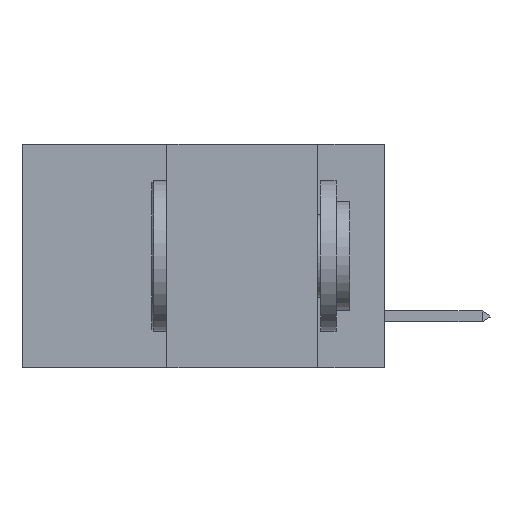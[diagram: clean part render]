
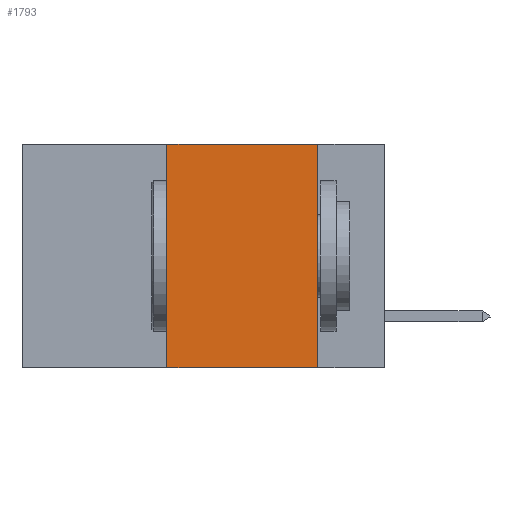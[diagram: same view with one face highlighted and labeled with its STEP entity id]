
A CAD part, left-side view. The second image highlights one B-rep face of the part: STEP entity #1793.
In plain terms, the highlighted planar face has unit normal (-1, 0, 0).
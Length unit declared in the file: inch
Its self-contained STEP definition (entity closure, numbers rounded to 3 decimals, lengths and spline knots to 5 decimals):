
#1087 = AXIS2_PLACEMENT_3D ( 'NONE', #40869, #5849, #6008 ) ;
#1793 = ADVANCED_FACE ( 'NONE', ( #32302 ), #26774, .F. ) ;
#3799 = ORIENTED_EDGE ( 'NONE', *, *, #31050, .F. ) ;
#4231 = CARTESIAN_POINT ( 'NONE',  ( 0., 0.11, 0. ) ) ;
#5849 = DIRECTION ( 'NONE',  ( 1., 0., 0. ) ) ;
#6008 = DIRECTION ( 'NONE',  ( 0., 0., -1. ) ) ;
#9077 = EDGE_CURVE ( 'NONE', #22593, #15512, #11155, .T. ) ;
#10060 = LINE ( 'NONE', #16562, #19958 ) ;
#10711 = CARTESIAN_POINT ( 'NONE',  ( 0., 0.11, 0. ) ) ;
#10916 = ORIENTED_EDGE ( 'NONE', *, *, #9077, .F. ) ;
#11155 = LINE ( 'NONE', #17633, #39161 ) ;
#11325 = EDGE_CURVE ( 'NONE', #22593, #28949, #37091, .T. ) ;
#12124 = CARTESIAN_POINT ( 'NONE',  ( 0., 0.6, -0.37 ) ) ;
#12351 = VECTOR ( 'NONE', #33935, 39.37008 ) ;
#13168 = LINE ( 'NONE', #4231, #26885 ) ;
#15512 = VERTEX_POINT ( 'NONE', #18373 ) ;
#16562 = CARTESIAN_POINT ( 'NONE',  ( 0., 0.6, 0. ) ) ;
#17633 = CARTESIAN_POINT ( 'NONE',  ( 0., 0.36, 0. ) ) ;
#18373 = CARTESIAN_POINT ( 'NONE',  ( 0., 0.36, 0. ) ) ;
#18925 = CARTESIAN_POINT ( 'NONE',  ( 0., 0.11, -0.37 ) ) ;
#19958 = VECTOR ( 'NONE', #30417, 39.37008 ) ;
#21933 = DIRECTION ( 'NONE',  ( 0., 0., -1. ) ) ;
#22593 = VERTEX_POINT ( 'NONE', #24009 ) ;
#24009 = CARTESIAN_POINT ( 'NONE',  ( 0., 0.36, -0.37 ) ) ;
#25228 = ORIENTED_EDGE ( 'NONE', *, *, #36069, .F. ) ;
#26774 = PLANE ( 'NONE',  #1087 ) ;
#26885 = VECTOR ( 'NONE', #21933, 39.37008 ) ;
#28657 = DIRECTION ( 'NONE',  ( 0., 0., 1. ) ) ;
#28776 = EDGE_LOOP ( 'NONE', ( #3799, #25228, #10916, #38512 ) ) ;
#28949 = VERTEX_POINT ( 'NONE', #18925 ) ;
#30417 = DIRECTION ( 'NONE',  ( 0., -1., 0. ) ) ;
#31050 = EDGE_CURVE ( 'NONE', #31366, #28949, #13168, .T. ) ;
#31366 = VERTEX_POINT ( 'NONE', #10711 ) ;
#32302 = FACE_OUTER_BOUND ( 'NONE', #28776, .T. ) ;
#33935 = DIRECTION ( 'NONE',  ( 0., -1., 0. ) ) ;
#36069 = EDGE_CURVE ( 'NONE', #15512, #31366, #10060, .T. ) ;
#37091 = LINE ( 'NONE', #12124, #12351 ) ;
#38512 = ORIENTED_EDGE ( 'NONE', *, *, #11325, .T. ) ;
#39161 = VECTOR ( 'NONE', #28657, 39.37008 ) ;
#40869 = CARTESIAN_POINT ( 'NONE',  ( 0., 0.6, 0. ) ) ;
